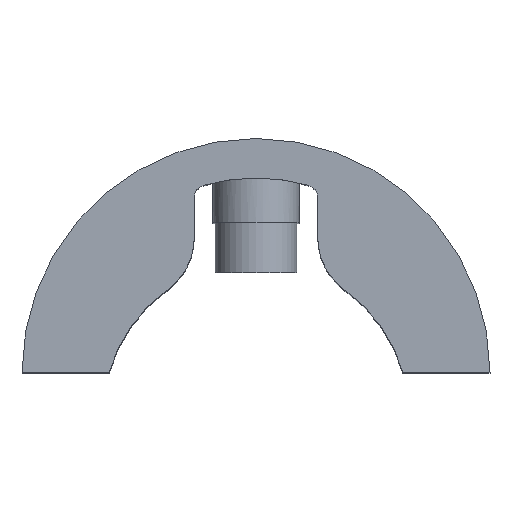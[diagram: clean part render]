
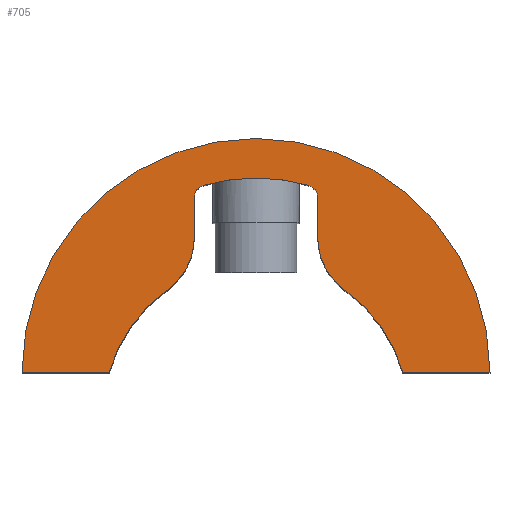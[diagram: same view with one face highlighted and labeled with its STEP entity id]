
A CAD part, top view. The second image highlights one B-rep face of the part: STEP entity #705.
In plain terms, the highlighted planar face has unit normal (0, 0, 1).
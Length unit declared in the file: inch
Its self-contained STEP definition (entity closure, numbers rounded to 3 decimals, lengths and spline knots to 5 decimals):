
#2 = DIRECTION ( 'NONE',  ( 0., 0., 1. ) ) ;
#11 = CARTESIAN_POINT ( 'NONE',  ( 0.56509, 0.1607, -1. ) ) ;
#13 = CARTESIAN_POINT ( 'NONE',  ( -0.9, 0.1607, -1. ) ) ;
#17 = CARTESIAN_POINT ( 'NONE',  ( 0.2375, 0., -1. ) ) ;
#50 = DIRECTION ( 'NONE',  ( 1., 0., 0. ) ) ;
#57 = CARTESIAN_POINT ( 'NONE',  ( 0.4875, 0.68099, -1. ) ) ;
#72 = AXIS2_PLACEMENT_3D ( 'NONE', #57, #361, #291 ) ;
#101 = CARTESIAN_POINT ( 'NONE',  ( -0.2375, 0.83562, -1. ) ) ;
#129 = ORIENTED_EDGE ( 'NONE', *, *, #292, .T. ) ;
#155 = CARTESIAN_POINT ( 'NONE',  ( 0.20337, 0.88074, -1. ) ) ;
#158 = DIRECTION ( 'NONE',  ( 0., -1., 0. ) ) ;
#165 = DIRECTION ( 'NONE',  ( 1., 0., 0. ) ) ;
#167 = DIRECTION ( 'NONE',  ( 0., 0., 1. ) ) ;
#168 = CARTESIAN_POINT ( 'NONE',  ( 0.19062, 0.83562, -1. ) ) ;
#184 = VERTEX_POINT ( 'NONE', #724 ) ;
#205 = EDGE_CURVE ( 'NONE', #791, #184, #550, .T. ) ;
#214 = AXIS2_PLACEMENT_3D ( 'NONE', #259, #222, #165 ) ;
#222 = DIRECTION ( 'NONE',  ( 0., 0., 1. ) ) ;
#223 = CARTESIAN_POINT ( 'NONE',  ( 0., 0., -1. ) ) ;
#226 = AXIS2_PLACEMENT_3D ( 'NONE', #635, #167, #726 ) ;
#236 = CARTESIAN_POINT ( 'NONE',  ( 0., 0., -1. ) ) ;
#254 = AXIS2_PLACEMENT_3D ( 'NONE', #223, #2, #897 ) ;
#259 = CARTESIAN_POINT ( 'NONE',  ( 0., 0., -1. ) ) ;
#264 = DIRECTION ( 'NONE',  ( 0., 0., 1. ) ) ;
#266 = CARTESIAN_POINT ( 'NONE',  ( -0.19062, 0.83562, -1. ) ) ;
#281 = PLANE ( 'NONE',  #254 ) ;
#288 = DIRECTION ( 'NONE',  ( 1., 0., 0. ) ) ;
#291 = DIRECTION ( 'NONE',  ( 1., 0., 0. ) ) ;
#292 = EDGE_CURVE ( 'NONE', #573, #184, #521, .T. ) ;
#303 = DIRECTION ( 'NONE',  ( 1., 0., 0. ) ) ;
#317 = CIRCLE ( 'NONE', #845, 0.9 ) ;
#327 = AXIS2_PLACEMENT_3D ( 'NONE', #789, #264, #875 ) ;
#329 = VECTOR ( 'NONE', #866, 39.37008 ) ;
#336 = DIRECTION ( 'NONE',  ( -1., 0., 0. ) ) ;
#338 = LINE ( 'NONE', #606, #329 ) ;
#341 = EDGE_CURVE ( 'NONE', #573, #691, #502, .T. ) ;
#348 = CIRCLE ( 'NONE', #431, 0.5875 ) ;
#352 = DIRECTION ( 'NONE',  ( 1., 0., 0. ) ) ;
#361 = DIRECTION ( 'NONE',  ( 0., 0., 1. ) ) ;
#370 = CARTESIAN_POINT ( 'NONE',  ( -0.2375, 0.68099, -1. ) ) ;
#395 = CIRCLE ( 'NONE', #226, 0.25 ) ;
#402 = FACE_OUTER_BOUND ( 'NONE', #879, .T. ) ;
#410 = VECTOR ( 'NONE', #158, 39.37008 ) ;
#411 = LINE ( 'NONE', #449, #410 ) ;
#414 = EDGE_CURVE ( 'NONE', #691, #611, #489, .T. ) ;
#423 = CIRCLE ( 'NONE', #633, 0.04688 ) ;
#431 = AXIS2_PLACEMENT_3D ( 'NONE', #236, #828, #303 ) ;
#432 = CIRCLE ( 'NONE', #327, 0.7482 ) ;
#441 = DIRECTION ( 'NONE',  ( 0., 0., 1. ) ) ;
#445 = VECTOR ( 'NONE', #336, 39.37008 ) ;
#446 = LINE ( 'NONE', #655, #445 ) ;
#449 = CARTESIAN_POINT ( 'NONE',  ( -0.2375, 0., -1. ) ) ;
#472 = CARTESIAN_POINT ( 'NONE',  ( -0.34198, 0.47771, -1. ) ) ;
#478 = EDGE_CURVE ( 'NONE', #927, #841, #446, .T. ) ;
#479 = DIRECTION ( 'NONE',  ( 0., 1., 0. ) ) ;
#489 = CIRCLE ( 'NONE', #657, 0.04687 ) ;
#500 = VECTOR ( 'NONE', #479, 39.37008 ) ;
#502 = LINE ( 'NONE', #17, #500 ) ;
#506 = CARTESIAN_POINT ( 'NONE',  ( -0.20337, 0.88074, -1. ) ) ;
#521 = CIRCLE ( 'NONE', #72, 0.25 ) ;
#527 = CARTESIAN_POINT ( 'NONE',  ( 0.2375, 0.83562, -1. ) ) ;
#534 = EDGE_CURVE ( 'NONE', #611, #874, #432, .T. ) ;
#550 = CIRCLE ( 'NONE', #214, 0.5875 ) ;
#573 = VERTEX_POINT ( 'NONE', #609 ) ;
#593 = EDGE_CURVE ( 'NONE', #874, #937, #423, .T. ) ;
#606 = CARTESIAN_POINT ( 'NONE',  ( 0., 0.1607, -1. ) ) ;
#609 = CARTESIAN_POINT ( 'NONE',  ( 0.2375, 0.68099, -1. ) ) ;
#611 = VERTEX_POINT ( 'NONE', #155 ) ;
#633 = AXIS2_PLACEMENT_3D ( 'NONE', #266, #877, #352 ) ;
#635 = CARTESIAN_POINT ( 'NONE',  ( -0.4875, 0.68099, -1. ) ) ;
#655 = CARTESIAN_POINT ( 'NONE',  ( 0., 0.1607, -1. ) ) ;
#657 = AXIS2_PLACEMENT_3D ( 'NONE', #168, #812, #288 ) ;
#665 = EDGE_CURVE ( 'NONE', #937, #739, #411, .T. ) ;
#691 = VERTEX_POINT ( 'NONE', #527 ) ;
#705 = ADVANCED_FACE ( 'NONE', ( #402 ), #281, .T. ) ;
#718 = EDGE_CURVE ( 'NONE', #864, #739, #395, .T. ) ;
#724 = CARTESIAN_POINT ( 'NONE',  ( 0.34198, 0.47771, -1. ) ) ;
#726 = DIRECTION ( 'NONE',  ( 1., 0., 0. ) ) ;
#739 = VERTEX_POINT ( 'NONE', #370 ) ;
#753 = VERTEX_POINT ( 'NONE', #811 ) ;
#758 = ORIENTED_EDGE ( 'NONE', *, *, #341, .F. ) ;
#787 = CARTESIAN_POINT ( 'NONE',  ( -0.56509, 0.1607, -1. ) ) ;
#789 = CARTESIAN_POINT ( 'NONE',  ( 0., 0.1607, -1. ) ) ;
#791 = VERTEX_POINT ( 'NONE', #11 ) ;
#795 = ORIENTED_EDGE ( 'NONE', *, *, #947, .T. ) ;
#811 = CARTESIAN_POINT ( 'NONE',  ( 0.9, 0.1607, -1. ) ) ;
#812 = DIRECTION ( 'NONE',  ( 0., 0., 1. ) ) ;
#819 = ORIENTED_EDGE ( 'NONE', *, *, #414, .F. ) ;
#823 = ORIENTED_EDGE ( 'NONE', *, *, #896, .F. ) ;
#828 = DIRECTION ( 'NONE',  ( 0., 0., 1. ) ) ;
#840 = EDGE_CURVE ( 'NONE', #864, #927, #348, .T. ) ;
#841 = VERTEX_POINT ( 'NONE', #13 ) ;
#845 = AXIS2_PLACEMENT_3D ( 'NONE', #963, #441, #50 ) ;
#864 = VERTEX_POINT ( 'NONE', #472 ) ;
#866 = DIRECTION ( 'NONE',  ( -1., 0., 0. ) ) ;
#868 = ORIENTED_EDGE ( 'NONE', *, *, #593, .F. ) ;
#874 = VERTEX_POINT ( 'NONE', #506 ) ;
#875 = DIRECTION ( 'NONE',  ( 1., 0., 0. ) ) ;
#877 = DIRECTION ( 'NONE',  ( 0., 0., 1. ) ) ;
#879 = EDGE_LOOP ( 'NONE', ( #823, #795, #933, #902, #941, #940, #868, #904, #819, #758, #129, #961 ) ) ;
#896 = EDGE_CURVE ( 'NONE', #753, #791, #338, .T. ) ;
#897 = DIRECTION ( 'NONE',  ( 1., 0., 0. ) ) ;
#902 = ORIENTED_EDGE ( 'NONE', *, *, #840, .F. ) ;
#904 = ORIENTED_EDGE ( 'NONE', *, *, #534, .F. ) ;
#927 = VERTEX_POINT ( 'NONE', #787 ) ;
#933 = ORIENTED_EDGE ( 'NONE', *, *, #478, .F. ) ;
#937 = VERTEX_POINT ( 'NONE', #101 ) ;
#940 = ORIENTED_EDGE ( 'NONE', *, *, #665, .F. ) ;
#941 = ORIENTED_EDGE ( 'NONE', *, *, #718, .T. ) ;
#947 = EDGE_CURVE ( 'NONE', #753, #841, #317, .T. ) ;
#961 = ORIENTED_EDGE ( 'NONE', *, *, #205, .F. ) ;
#963 = CARTESIAN_POINT ( 'NONE',  ( 0., 0.1607, -1. ) ) ;
